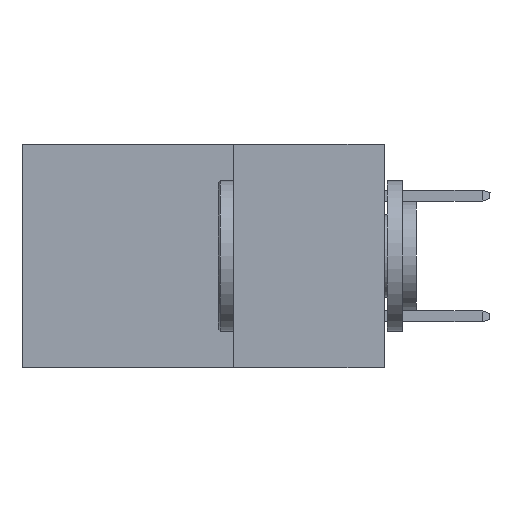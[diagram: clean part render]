
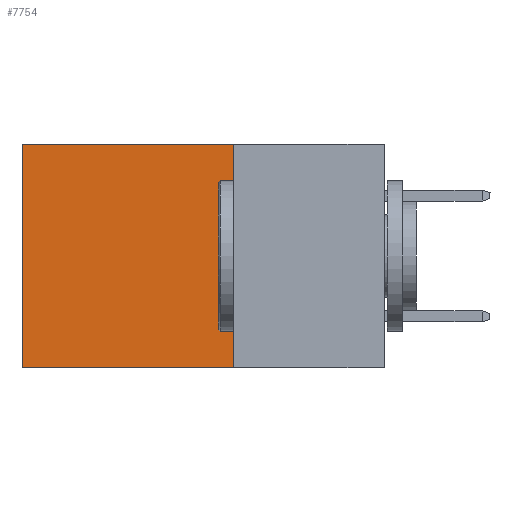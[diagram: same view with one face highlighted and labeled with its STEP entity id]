
A CAD part, left-side view. The second image highlights one B-rep face of the part: STEP entity #7754.
In plain terms, the highlighted planar face has unit normal (-1, 0, 0).
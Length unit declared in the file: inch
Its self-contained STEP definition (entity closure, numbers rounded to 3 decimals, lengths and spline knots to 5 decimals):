
#244 = VERTEX_POINT ( 'NONE', #1304 ) ;
#880 = LINE ( 'NONE', #10993, #1868 ) ;
#1187 = CARTESIAN_POINT ( 'NONE',  ( 0.298, 0.6, -0.37 ) ) ;
#1272 = FACE_OUTER_BOUND ( 'NONE', #9519, .T. ) ;
#1304 = CARTESIAN_POINT ( 'NONE',  ( 0.298, 0.25, 0. ) ) ;
#1506 = DIRECTION ( 'NONE',  ( 1., 0., 0. ) ) ;
#1868 = VECTOR ( 'NONE', #10857, 39.37008 ) ;
#2130 = VERTEX_POINT ( 'NONE', #9951 ) ;
#2638 = ORIENTED_EDGE ( 'NONE', *, *, #8454, .T. ) ;
#2645 = DIRECTION ( 'NONE',  ( 0., 0., -1. ) ) ;
#3002 = AXIS2_PLACEMENT_3D ( 'NONE', #6608, #1506, #2645 ) ;
#3677 = PLANE ( 'NONE',  #3002 ) ;
#3949 = ORIENTED_EDGE ( 'NONE', *, *, #11358, .T. ) ;
#4081 = DIRECTION ( 'NONE',  ( 0., 1., 0. ) ) ;
#4332 = EDGE_CURVE ( 'NONE', #7619, #9630, #12737, .T. ) ;
#5314 = EDGE_CURVE ( 'NONE', #244, #7619, #8851, .T. ) ;
#5792 = CARTESIAN_POINT ( 'NONE',  ( 0.298, 0.25, 0. ) ) ;
#6118 = CARTESIAN_POINT ( 'NONE',  ( 0.298, 0.25, -0.37 ) ) ;
#6453 = VECTOR ( 'NONE', #8824, 39.37008 ) ;
#6510 = VECTOR ( 'NONE', #12197, 39.37008 ) ;
#6608 = CARTESIAN_POINT ( 'NONE',  ( 0.298, 0.25, 0. ) ) ;
#6688 = LINE ( 'NONE', #12114, #6510 ) ;
#7619 = VERTEX_POINT ( 'NONE', #9619 ) ;
#7635 = ORIENTED_EDGE ( 'NONE', *, *, #5314, .F. ) ;
#7754 = ADVANCED_FACE ( 'NONE', ( #1272 ), #3677, .F. ) ;
#8454 = EDGE_CURVE ( 'NONE', #244, #2130, #880, .T. ) ;
#8824 = DIRECTION ( 'NONE',  ( 0., 0., -1. ) ) ;
#8851 = LINE ( 'NONE', #5792, #6453 ) ;
#9519 = EDGE_LOOP ( 'NONE', ( #3949, #11330, #7635, #2638 ) ) ;
#9619 = CARTESIAN_POINT ( 'NONE',  ( 0.298, 0.25, -0.37 ) ) ;
#9630 = VERTEX_POINT ( 'NONE', #1187 ) ;
#9951 = CARTESIAN_POINT ( 'NONE',  ( 0.298, 0.6, 0. ) ) ;
#10857 = DIRECTION ( 'NONE',  ( 0., 1., 0. ) ) ;
#10993 = CARTESIAN_POINT ( 'NONE',  ( 0.298, 0.25, 0. ) ) ;
#11162 = VECTOR ( 'NONE', #4081, 39.37008 ) ;
#11330 = ORIENTED_EDGE ( 'NONE', *, *, #4332, .F. ) ;
#11358 = EDGE_CURVE ( 'NONE', #2130, #9630, #6688, .T. ) ;
#12114 = CARTESIAN_POINT ( 'NONE',  ( 0.298, 0.6, 0. ) ) ;
#12197 = DIRECTION ( 'NONE',  ( 0., 0., -1. ) ) ;
#12737 = LINE ( 'NONE', #6118, #11162 ) ;
